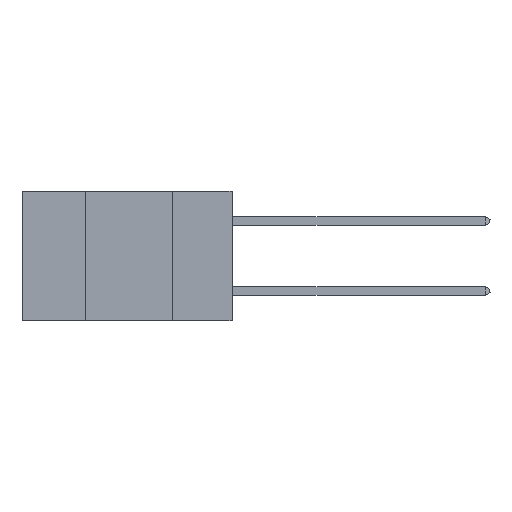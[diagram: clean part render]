
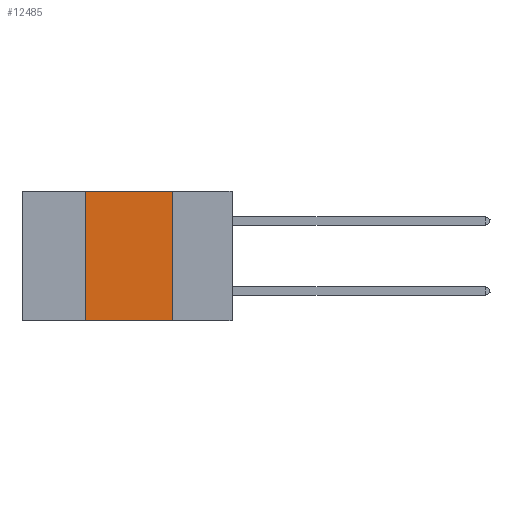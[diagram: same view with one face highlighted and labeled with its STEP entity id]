
A CAD part, left-side view. The second image highlights one B-rep face of the part: STEP entity #12485.
In plain terms, the highlighted planar face has unit normal (-1, 0, 0).
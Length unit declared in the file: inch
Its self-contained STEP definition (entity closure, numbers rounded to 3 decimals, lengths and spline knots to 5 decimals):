
#196 = VECTOR ( 'NONE', #4544, 39.37008 ) ;
#1762 = LINE ( 'NONE', #28337, #29634 ) ;
#1843 = CARTESIAN_POINT ( 'NONE',  ( 0., 0.42, 0. ) ) ;
#2132 = CARTESIAN_POINT ( 'NONE',  ( 0., 0.17, 0. ) ) ;
#3583 = DIRECTION ( 'NONE',  ( 0., 0., -1. ) ) ;
#4488 = DIRECTION ( 'NONE',  ( 0., -1., 0. ) ) ;
#4544 = DIRECTION ( 'NONE',  ( 0., 0., 1. ) ) ;
#7431 = ORIENTED_EDGE ( 'NONE', *, *, #18294, .F. ) ;
#10285 = VERTEX_POINT ( 'NONE', #17674 ) ;
#10546 = VERTEX_POINT ( 'NONE', #27000 ) ;
#11121 = VERTEX_POINT ( 'NONE', #2132 ) ;
#11316 = CARTESIAN_POINT ( 'NONE',  ( 0., 0.6, 0. ) ) ;
#12388 = CARTESIAN_POINT ( 'NONE',  ( 0., 0.17, -0.37 ) ) ;
#12485 = ADVANCED_FACE ( 'NONE', ( #30460 ), #29740, .F. ) ;
#12513 = VERTEX_POINT ( 'NONE', #12388 ) ;
#12578 = DIRECTION ( 'NONE',  ( 0., -1., 0. ) ) ;
#13551 = DIRECTION ( 'NONE',  ( 1., 0., 0. ) ) ;
#14471 = VECTOR ( 'NONE', #4488, 39.37008 ) ;
#17674 = CARTESIAN_POINT ( 'NONE',  ( 0., 0.42, 0. ) ) ;
#18278 = LINE ( 'NONE', #23669, #14471 ) ;
#18294 = EDGE_CURVE ( 'NONE', #10285, #11121, #1762, .T. ) ;
#20037 = CARTESIAN_POINT ( 'NONE',  ( 0., 0.17, 0. ) ) ;
#21231 = AXIS2_PLACEMENT_3D ( 'NONE', #11316, #13551, #32457 ) ;
#22648 = LINE ( 'NONE', #1843, #196 ) ;
#23669 = CARTESIAN_POINT ( 'NONE',  ( 0., 0.6, -0.37 ) ) ;
#25929 = LINE ( 'NONE', #20037, #26369 ) ;
#26369 = VECTOR ( 'NONE', #3583, 39.37008 ) ;
#26594 = ORIENTED_EDGE ( 'NONE', *, *, #34927, .F. ) ;
#26599 = ORIENTED_EDGE ( 'NONE', *, *, #30241, .T. ) ;
#27000 = CARTESIAN_POINT ( 'NONE',  ( 0., 0.42, -0.37 ) ) ;
#28337 = CARTESIAN_POINT ( 'NONE',  ( 0., 0.6, 0. ) ) ;
#29634 = VECTOR ( 'NONE', #12578, 39.37008 ) ;
#29740 = PLANE ( 'NONE',  #21231 ) ;
#29836 = EDGE_LOOP ( 'NONE', ( #31397, #7431, #26594, #26599 ) ) ;
#30241 = EDGE_CURVE ( 'NONE', #10546, #12513, #18278, .T. ) ;
#30460 = FACE_OUTER_BOUND ( 'NONE', #29836, .T. ) ;
#30663 = EDGE_CURVE ( 'NONE', #11121, #12513, #25929, .T. ) ;
#31397 = ORIENTED_EDGE ( 'NONE', *, *, #30663, .F. ) ;
#32457 = DIRECTION ( 'NONE',  ( 0., 0., -1. ) ) ;
#34927 = EDGE_CURVE ( 'NONE', #10546, #10285, #22648, .T. ) ;
